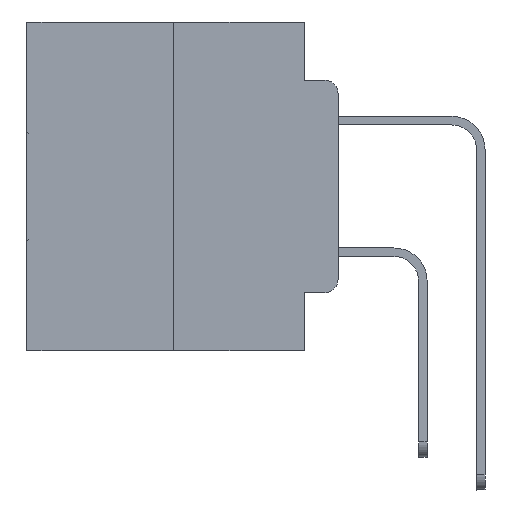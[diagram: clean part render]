
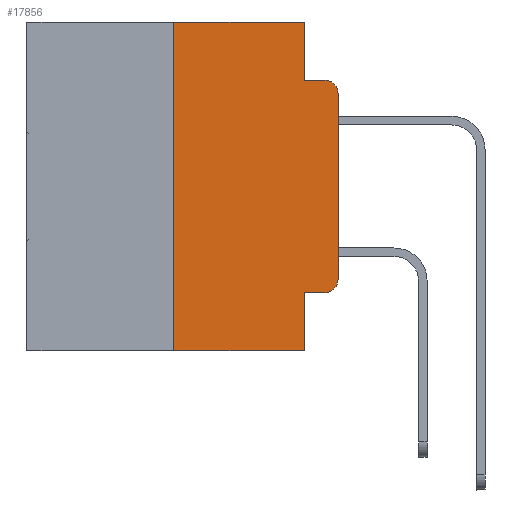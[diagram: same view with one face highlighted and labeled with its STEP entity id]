
A CAD part, left-side view. The second image highlights one B-rep face of the part: STEP entity #17856.
In plain terms, the highlighted planar face has unit normal (-1, 0, 0).
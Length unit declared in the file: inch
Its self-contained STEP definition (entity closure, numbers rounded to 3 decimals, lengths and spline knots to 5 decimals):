
#111 = VERTEX_POINT ( 'NONE', #11098 ) ;
#146 = DIRECTION ( 'NONE',  ( 0., -1., 0. ) ) ;
#457 = DIRECTION ( 'NONE',  ( 0., 0., -1. ) ) ;
#658 = VECTOR ( 'NONE', #3345, 39.37008 ) ;
#1616 = VECTOR ( 'NONE', #5018, 39.37008 ) ;
#1645 = DIRECTION ( 'NONE',  ( 0., -1., 0. ) ) ;
#2256 = ORIENTED_EDGE ( 'NONE', *, *, #23312, .T. ) ;
#2441 = DIRECTION ( 'NONE',  ( 1., 0., 0. ) ) ;
#2671 = ORIENTED_EDGE ( 'NONE', *, *, #21638, .T. ) ;
#2703 = ORIENTED_EDGE ( 'NONE', *, *, #3879, .T. ) ;
#3345 = DIRECTION ( 'NONE',  ( 0., 0., 1. ) ) ;
#3510 = ORIENTED_EDGE ( 'NONE', *, *, #10172, .F. ) ;
#3593 = VECTOR ( 'NONE', #1645, 39.37008 ) ;
#3879 = EDGE_CURVE ( 'NONE', #14887, #14778, #16756, .T. ) ;
#3904 = ORIENTED_EDGE ( 'NONE', *, *, #15031, .F. ) ;
#4700 = VERTEX_POINT ( 'NONE', #19266 ) ;
#5018 = DIRECTION ( 'NONE',  ( 0., -1., 0. ) ) ;
#5076 = VECTOR ( 'NONE', #457, 39.37008 ) ;
#5162 = EDGE_CURVE ( 'NONE', #4700, #27654, #13947, .T. ) ;
#5192 = CIRCLE ( 'NONE', #15190, 0.02 ) ;
#5519 = VERTEX_POINT ( 'NONE', #17736 ) ;
#6475 = DIRECTION ( 'NONE',  ( -1., 0., 0. ) ) ;
#6844 = EDGE_CURVE ( 'NONE', #20351, #4700, #30655, .T. ) ;
#7476 = CARTESIAN_POINT ( 'NONE',  ( 0., 0.25, -0.5 ) ) ;
#7583 = LINE ( 'NONE', #19739, #1616 ) ;
#7827 = CARTESIAN_POINT ( 'NONE',  ( 0., 0.473, 0. ) ) ;
#8201 = VECTOR ( 'NONE', #18091, 39.37008 ) ;
#8784 = CARTESIAN_POINT ( 'NONE',  ( 0., 0.02, -0.1085 ) ) ;
#10052 = CARTESIAN_POINT ( 'NONE',  ( 0., 0., -0.1085 ) ) ;
#10172 = EDGE_CURVE ( 'NONE', #20351, #14778, #21993, .T. ) ;
#10703 = CARTESIAN_POINT ( 'NONE',  ( 0., 0.051, 0. ) ) ;
#11098 = CARTESIAN_POINT ( 'NONE',  ( 0., 0.25, 0. ) ) ;
#11234 = AXIS2_PLACEMENT_3D ( 'NONE', #17315, #2441, #19765 ) ;
#11249 = DIRECTION ( 'NONE',  ( 0., 0., -1. ) ) ;
#11545 = DIRECTION ( 'NONE',  ( 0., 0., 1. ) ) ;
#11704 = ORIENTED_EDGE ( 'NONE', *, *, #6844, .T. ) ;
#11821 = CARTESIAN_POINT ( 'NONE',  ( 0., 0.051, 0. ) ) ;
#12701 = VERTEX_POINT ( 'NONE', #11821 ) ;
#12822 = ORIENTED_EDGE ( 'NONE', *, *, #22484, .F. ) ;
#13407 = EDGE_CURVE ( 'NONE', #14887, #111, #29028, .T. ) ;
#13947 = CIRCLE ( 'NONE', #23073, 0.02 ) ;
#14392 = CARTESIAN_POINT ( 'NONE',  ( 0., 0.051, -0.5 ) ) ;
#14778 = VERTEX_POINT ( 'NONE', #14392 ) ;
#14887 = VERTEX_POINT ( 'NONE', #7476 ) ;
#15031 = EDGE_CURVE ( 'NONE', #12701, #5519, #24687, .T. ) ;
#15190 = AXIS2_PLACEMENT_3D ( 'NONE', #8784, #25893, #11249 ) ;
#15582 = DIRECTION ( 'NONE',  ( 0., -1., 0. ) ) ;
#16756 = LINE ( 'NONE', #21484, #3593 ) ;
#17315 = CARTESIAN_POINT ( 'NONE',  ( 0., 0.473, 0. ) ) ;
#17736 = CARTESIAN_POINT ( 'NONE',  ( 0., 0.051, -0.0885 ) ) ;
#17856 = ADVANCED_FACE ( 'NONE', ( #27901 ), #29459, .F. ) ;
#18091 = DIRECTION ( 'NONE',  ( 0., 0., -1. ) ) ;
#18350 = EDGE_CURVE ( 'NONE', #5519, #29310, #7583, .T. ) ;
#18493 = CARTESIAN_POINT ( 'NONE',  ( 0., 0.051, -0.4115 ) ) ;
#19266 = CARTESIAN_POINT ( 'NONE',  ( 0., 0.02, -0.4115 ) ) ;
#19720 = ORIENTED_EDGE ( 'NONE', *, *, #18350, .F. ) ;
#19739 = CARTESIAN_POINT ( 'NONE',  ( 0., 0.051, -0.0885 ) ) ;
#19765 = DIRECTION ( 'NONE',  ( 0., 0., -1. ) ) ;
#20351 = VERTEX_POINT ( 'NONE', #18493 ) ;
#21171 = CARTESIAN_POINT ( 'NONE',  ( 0., 0.02, -0.3915 ) ) ;
#21293 = CARTESIAN_POINT ( 'NONE',  ( 0., 0.25, 0. ) ) ;
#21484 = CARTESIAN_POINT ( 'NONE',  ( 0., 0.473, -0.5 ) ) ;
#21638 = EDGE_CURVE ( 'NONE', #29197, #29310, #5192, .T. ) ;
#21993 = LINE ( 'NONE', #10703, #8201 ) ;
#22484 = EDGE_CURVE ( 'NONE', #111, #12701, #31156, .T. ) ;
#22582 = VECTOR ( 'NONE', #11545, 39.37008 ) ;
#22662 = CARTESIAN_POINT ( 'NONE',  ( 0., 0.02, -0.0885 ) ) ;
#22914 = CARTESIAN_POINT ( 'NONE',  ( 0., 0.051, -0.4115 ) ) ;
#23073 = AXIS2_PLACEMENT_3D ( 'NONE', #21171, #6475, #23653 ) ;
#23312 = EDGE_CURVE ( 'NONE', #27654, #29197, #26947, .T. ) ;
#23653 = DIRECTION ( 'NONE',  ( 0., 0., -1. ) ) ;
#24241 = VECTOR ( 'NONE', #15582, 39.37008 ) ;
#24687 = LINE ( 'NONE', #30002, #5076 ) ;
#24968 = EDGE_LOOP ( 'NONE', ( #2256, #2671, #19720, #3904, #12822, #25865, #2703, #3510, #11704, #27777 ) ) ;
#25865 = ORIENTED_EDGE ( 'NONE', *, *, #13407, .F. ) ;
#25893 = DIRECTION ( 'NONE',  ( -1., 0., 0. ) ) ;
#26947 = LINE ( 'NONE', #27874, #658 ) ;
#27467 = CARTESIAN_POINT ( 'NONE',  ( 0., 0., -0.3915 ) ) ;
#27654 = VERTEX_POINT ( 'NONE', #27467 ) ;
#27777 = ORIENTED_EDGE ( 'NONE', *, *, #5162, .T. ) ;
#27874 = CARTESIAN_POINT ( 'NONE',  ( 0., 0., 0. ) ) ;
#27901 = FACE_OUTER_BOUND ( 'NONE', #24968, .T. ) ;
#29028 = LINE ( 'NONE', #21293, #22582 ) ;
#29197 = VERTEX_POINT ( 'NONE', #10052 ) ;
#29310 = VERTEX_POINT ( 'NONE', #22662 ) ;
#29459 = PLANE ( 'NONE',  #11234 ) ;
#29659 = VECTOR ( 'NONE', #146, 39.37008 ) ;
#30002 = CARTESIAN_POINT ( 'NONE',  ( 0., 0.051, 0. ) ) ;
#30655 = LINE ( 'NONE', #22914, #24241 ) ;
#31156 = LINE ( 'NONE', #7827, #29659 ) ;
